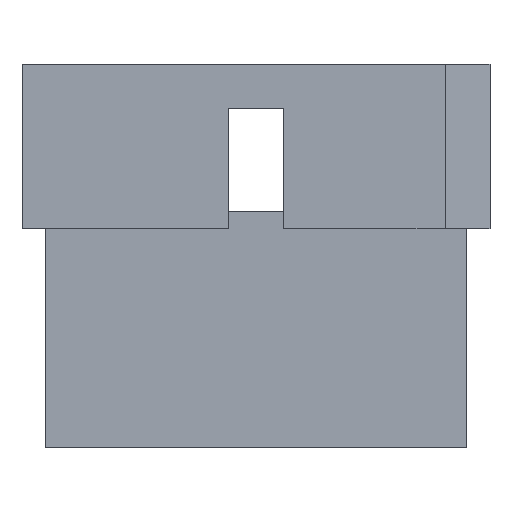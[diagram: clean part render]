
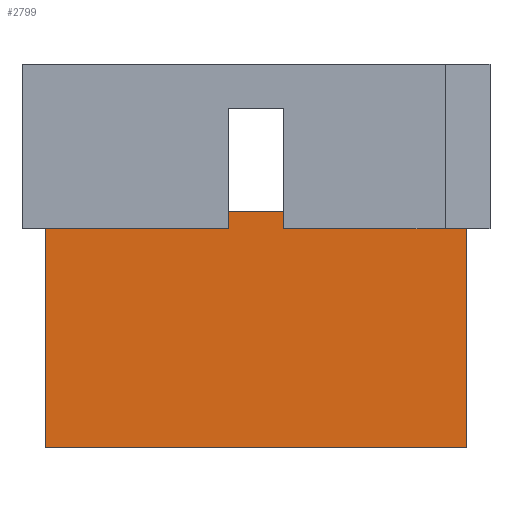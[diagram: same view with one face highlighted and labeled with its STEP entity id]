
A CAD part, top view. The second image highlights one B-rep face of the part: STEP entity #2799.
In plain terms, the highlighted planar face has unit normal (0, 0, 1).
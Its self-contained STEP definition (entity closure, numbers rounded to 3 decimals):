
#4 = LINE ( 'NONE', #649, #5116 ) ;
#74 = CARTESIAN_POINT ( 'NONE',  ( 8.306, 1.016, 2.54 ) ) ;
#168 = VERTEX_POINT ( 'NONE', #74 ) ;
#170 = CARTESIAN_POINT ( 'NONE',  ( -2.324, -12.7, 2.54 ) ) ;
#181 = VERTEX_POINT ( 'NONE', #656 ) ;
#502 = CARTESIAN_POINT ( 'NONE',  ( -2.324, -12.7, 2.54 ) ) ;
#649 = CARTESIAN_POINT ( 'NONE',  ( -2.324, 0., 2.54 ) ) ;
#656 = CARTESIAN_POINT ( 'NONE',  ( 11.506, 1.016, 2.54 ) ) ;
#673 = LINE ( 'NONE', #5953, #5591 ) ;
#741 = DIRECTION ( 'NONE',  ( 1., 0., 0. ) ) ;
#842 = FACE_OUTER_BOUND ( 'NONE', #4414, .T. ) ;
#911 = CARTESIAN_POINT ( 'NONE',  ( 11.506, 0., 2.54 ) ) ;
#981 = LINE ( 'NONE', #2800, #2630 ) ;
#1086 = VECTOR ( 'NONE', #4012, 1000. ) ;
#1104 = ORIENTED_EDGE ( 'NONE', *, *, #4303, .F. ) ;
#1326 = VERTEX_POINT ( 'NONE', #1694 ) ;
#1349 = AXIS2_PLACEMENT_3D ( 'NONE', #2649, #2129, #5541 ) ;
#1471 = ORIENTED_EDGE ( 'NONE', *, *, #5424, .T. ) ;
#1694 = CARTESIAN_POINT ( 'NONE',  ( 22.136, -12.7, 2.54 ) ) ;
#1793 = VECTOR ( 'NONE', #1996, 1000. ) ;
#1879 = CARTESIAN_POINT ( 'NONE',  ( 0., 1.016, 2.54 ) ) ;
#1993 = ORIENTED_EDGE ( 'NONE', *, *, #2152, .F. ) ;
#1994 = VERTEX_POINT ( 'NONE', #6193 ) ;
#1996 = DIRECTION ( 'NONE',  ( 1., 0., 0. ) ) ;
#2117 = VERTEX_POINT ( 'NONE', #911 ) ;
#2129 = DIRECTION ( 'NONE',  ( 0., 0., 1. ) ) ;
#2152 = EDGE_CURVE ( 'NONE', #168, #181, #3095, .T. ) ;
#2248 = ORIENTED_EDGE ( 'NONE', *, *, #3601, .T. ) ;
#2267 = VERTEX_POINT ( 'NONE', #502 ) ;
#2630 = VECTOR ( 'NONE', #5347, 1000. ) ;
#2649 = CARTESIAN_POINT ( 'NONE',  ( -2.324, -12.7, 2.54 ) ) ;
#2669 = EDGE_CURVE ( 'NONE', #168, #5453, #5908, .T. ) ;
#2799 = ADVANCED_FACE ( 'NONE', ( #842 ), #5632, .T. ) ;
#2800 = CARTESIAN_POINT ( 'NONE',  ( 22.136, -12.7, 2.54 ) ) ;
#2816 = EDGE_CURVE ( 'NONE', #1994, #5453, #4019, .T. ) ;
#2905 = EDGE_CURVE ( 'NONE', #2267, #1326, #3084, .T. ) ;
#3084 = LINE ( 'NONE', #4675, #3239 ) ;
#3095 = LINE ( 'NONE', #1879, #1793 ) ;
#3113 = DIRECTION ( 'NONE',  ( 0., 1., 0. ) ) ;
#3239 = VECTOR ( 'NONE', #741, 1000. ) ;
#3286 = CARTESIAN_POINT ( 'NONE',  ( 8.306, 0., 2.54 ) ) ;
#3400 = ORIENTED_EDGE ( 'NONE', *, *, #2669, .T. ) ;
#3495 = ORIENTED_EDGE ( 'NONE', *, *, #3680, .F. ) ;
#3540 = CARTESIAN_POINT ( 'NONE',  ( -2.324, 0., 2.54 ) ) ;
#3601 = EDGE_CURVE ( 'NONE', #2117, #181, #673, .T. ) ;
#3680 = EDGE_CURVE ( 'NONE', #2117, #6298, #4, .T. ) ;
#3891 = LINE ( 'NONE', #170, #6091 ) ;
#4012 = DIRECTION ( 'NONE',  ( 0., -1., 0. ) ) ;
#4019 = LINE ( 'NONE', #3540, #5364 ) ;
#4074 = DIRECTION ( 'NONE',  ( 1., 0., 0. ) ) ;
#4248 = CARTESIAN_POINT ( 'NONE',  ( 22.136, 0., 2.54 ) ) ;
#4303 = EDGE_CURVE ( 'NONE', #2267, #1994, #3891, .T. ) ;
#4414 = EDGE_LOOP ( 'NONE', ( #4515, #1104, #4512, #1471, #3495, #2248, #1993, #3400 ) ) ;
#4512 = ORIENTED_EDGE ( 'NONE', *, *, #2905, .T. ) ;
#4515 = ORIENTED_EDGE ( 'NONE', *, *, #2816, .F. ) ;
#4675 = CARTESIAN_POINT ( 'NONE',  ( -2.324, -12.7, 2.54 ) ) ;
#5008 = CARTESIAN_POINT ( 'NONE',  ( 8.306, 6.985, 2.54 ) ) ;
#5097 = DIRECTION ( 'NONE',  ( 1., 0., 0. ) ) ;
#5116 = VECTOR ( 'NONE', #4074, 1000. ) ;
#5347 = DIRECTION ( 'NONE',  ( 0., 1., 0. ) ) ;
#5364 = VECTOR ( 'NONE', #5097, 1000. ) ;
#5424 = EDGE_CURVE ( 'NONE', #1326, #6298, #981, .T. ) ;
#5453 = VERTEX_POINT ( 'NONE', #3286 ) ;
#5541 = DIRECTION ( 'NONE',  ( 1., 0., 0. ) ) ;
#5591 = VECTOR ( 'NONE', #6373, 1000. ) ;
#5632 = PLANE ( 'NONE',  #1349 ) ;
#5908 = LINE ( 'NONE', #5008, #1086 ) ;
#5953 = CARTESIAN_POINT ( 'NONE',  ( 11.506, 6.985, 2.54 ) ) ;
#6091 = VECTOR ( 'NONE', #3113, 1000. ) ;
#6193 = CARTESIAN_POINT ( 'NONE',  ( -2.324, 0., 2.54 ) ) ;
#6298 = VERTEX_POINT ( 'NONE', #4248 ) ;
#6373 = DIRECTION ( 'NONE',  ( 0., 1., 0. ) ) ;
